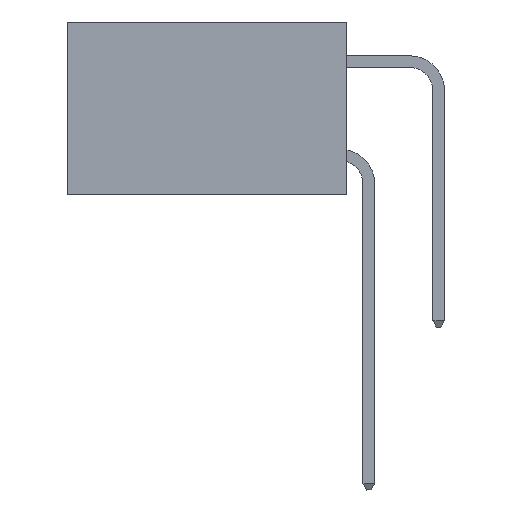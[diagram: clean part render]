
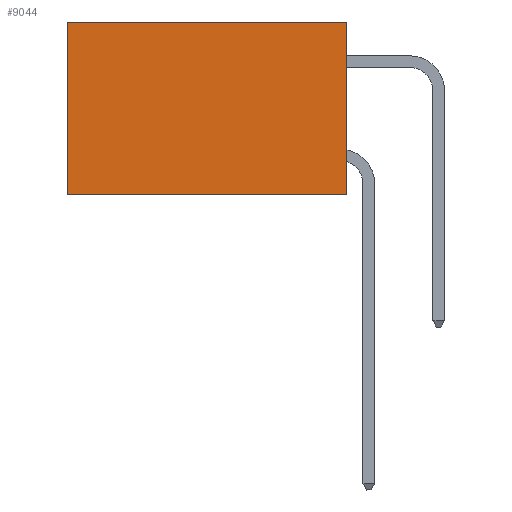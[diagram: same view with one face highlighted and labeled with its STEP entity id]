
A CAD part, left-side view. The second image highlights one B-rep face of the part: STEP entity #9044.
In plain terms, the highlighted planar face has unit normal (-1, 0, 0).
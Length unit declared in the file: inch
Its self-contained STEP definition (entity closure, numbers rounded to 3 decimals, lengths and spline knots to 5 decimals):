
#13 = DIRECTION ( 'NONE',  ( 0., 0., -1. ) ) ;
#203 = LINE ( 'NONE', #1280, #10776 ) ;
#530 = AXIS2_PLACEMENT_3D ( 'NONE', #7525, #624, #6412 ) ;
#624 = DIRECTION ( 'NONE',  ( 1., 0., 0. ) ) ;
#646 = DIRECTION ( 'NONE',  ( 0., 0., -1. ) ) ;
#1280 = CARTESIAN_POINT ( 'NONE',  ( 0.2875, 0., -0.37 ) ) ;
#1367 = CARTESIAN_POINT ( 'NONE',  ( 0.2875, 0., 0. ) ) ;
#1582 = FACE_OUTER_BOUND ( 'NONE', #14712, .T. ) ;
#1605 = EDGE_CURVE ( 'NONE', #12987, #12055, #12672, .T. ) ;
#1973 = CARTESIAN_POINT ( 'NONE',  ( 0.2875, 0., -0.37 ) ) ;
#2627 = DIRECTION ( 'NONE',  ( 0., 1., 0. ) ) ;
#4705 = VECTOR ( 'NONE', #13, 39.37008 ) ;
#5061 = EDGE_CURVE ( 'NONE', #12309, #11108, #203, .T. ) ;
#5379 = EDGE_CURVE ( 'NONE', #12987, #12309, #13089, .T. ) ;
#5509 = ORIENTED_EDGE ( 'NONE', *, *, #1605, .T. ) ;
#6336 = LINE ( 'NONE', #6894, #4705 ) ;
#6412 = DIRECTION ( 'NONE',  ( 0., 0., -1. ) ) ;
#6483 = CARTESIAN_POINT ( 'NONE',  ( 0.2875, 0., 0. ) ) ;
#6894 = CARTESIAN_POINT ( 'NONE',  ( 0.2875, 0.6, 0. ) ) ;
#6914 = DIRECTION ( 'NONE',  ( 0., 1., 0. ) ) ;
#6964 = ORIENTED_EDGE ( 'NONE', *, *, #5379, .F. ) ;
#7296 = ORIENTED_EDGE ( 'NONE', *, *, #12472, .T. ) ;
#7525 = CARTESIAN_POINT ( 'NONE',  ( 0.2875, 0., 0. ) ) ;
#7741 = VECTOR ( 'NONE', #646, 39.37008 ) ;
#8947 = ORIENTED_EDGE ( 'NONE', *, *, #5061, .F. ) ;
#9044 = ADVANCED_FACE ( 'NONE', ( #1582 ), #14548, .F. ) ;
#9117 = VECTOR ( 'NONE', #2627, 39.37008 ) ;
#10776 = VECTOR ( 'NONE', #6914, 39.37008 ) ;
#11108 = VERTEX_POINT ( 'NONE', #12603 ) ;
#12055 = VERTEX_POINT ( 'NONE', #13463 ) ;
#12309 = VERTEX_POINT ( 'NONE', #1973 ) ;
#12472 = EDGE_CURVE ( 'NONE', #12055, #11108, #6336, .T. ) ;
#12603 = CARTESIAN_POINT ( 'NONE',  ( 0.2875, 0.6, -0.37 ) ) ;
#12672 = LINE ( 'NONE', #12990, #9117 ) ;
#12987 = VERTEX_POINT ( 'NONE', #1367 ) ;
#12990 = CARTESIAN_POINT ( 'NONE',  ( 0.2875, 0., 0. ) ) ;
#13089 = LINE ( 'NONE', #6483, #7741 ) ;
#13463 = CARTESIAN_POINT ( 'NONE',  ( 0.2875, 0.6, 0. ) ) ;
#14548 = PLANE ( 'NONE',  #530 ) ;
#14712 = EDGE_LOOP ( 'NONE', ( #7296, #8947, #6964, #5509 ) ) ;
